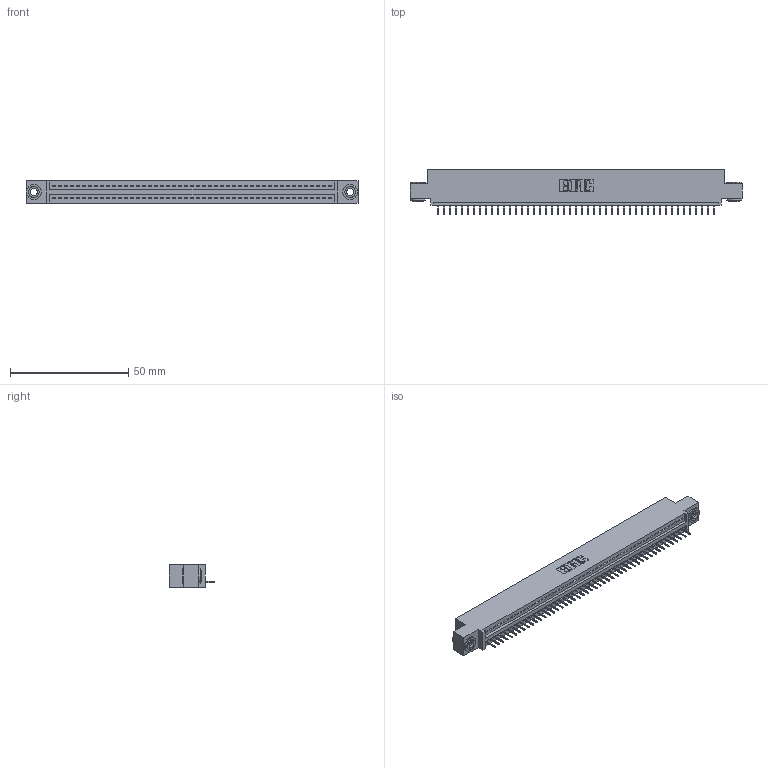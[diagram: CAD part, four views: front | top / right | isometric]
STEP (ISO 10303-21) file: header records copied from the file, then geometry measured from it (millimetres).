
FILE_DESCRIPTION (( 'STEP AP203' ), '1' );
FILE_NAME ('395-047-524-403.STEP', '2019-10-22T23:24:19', ( '' ), ( '' ), 'SwSTEP 2.0', 'SolidWorks 2016', '' );
FILE_SCHEMA (( 'CONFIG_CONTROL_DESIGN' ));
Length unit declared in the file: inch
Products named in the file (4): 395-047-524-403; 345-250-002_345-250-002-102; 345-292-001_345-293-124; 345 Part_0.110 Offset - 0.156 Dia-TH
Assembly tree (50 placements, depth 2):
  395-047-524-403
    345 Part_0.110 Offset - 0.156 Dia-TH
    345-292-001_345-293-124  x47
    345-250-002_345-250-002-102  x2
Bounding box: 140.59 x 19.35 x 9.4 mm (x, y, z)
Volume: 13154.6 mm3; surface area: 17252 mm2
Topology: 50 solids, 50 shells, 3082 faces, 8889 edges, 5734 vertices
Faces by surface type: plane 2256, cylinder 818, cone 8
Entity records: 35556 total; most frequent: CARTESIAN_POINT 6136, ORIENTED_EDGE 6110, DIRECTION 5383, EDGE_CURVE 3055, VECTOR 2715, LINE 2715, VERTEX_POINT 2030, AXIS2_PLACEMENT_3D 1334
